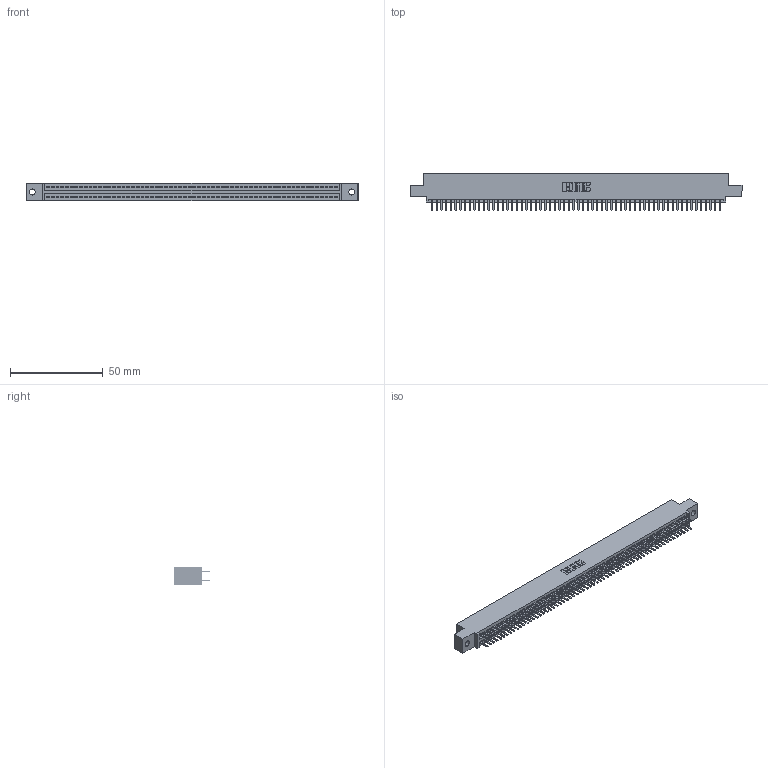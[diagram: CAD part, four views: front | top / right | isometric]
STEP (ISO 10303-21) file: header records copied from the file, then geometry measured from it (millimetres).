
FILE_DESCRIPTION (( 'STEP AP203' ), '1' );
FILE_NAME ('395-124-520-502.STEP', '2018-12-03T21:40:19', ( '' ), ( '' ), 'SwSTEP 2.0', 'SolidWorks 2016', '' );
FILE_SCHEMA (( 'CONFIG_CONTROL_DESIGN' ));
Length unit declared in the file: inch
Products named in the file (3): 395-124-520-502; 345-292-001_345-293-120; 345 Part_0.110 Offset - 0.128 Dia
Assembly tree (125 placements, depth 2):
  395-124-520-502
    345 Part_0.110 Offset - 0.128 Dia
    345-292-001_345-293-120  x124
Bounding box: 178.69 x 19.68 x 9.4 mm (x, y, z)
Volume: 17379.1 mm3; surface area: 25780.8 mm2
Topology: 125 solids, 125 shells, 6826 faces, 19821 edges, 12882 vertices
Faces by surface type: plane 4424, cylinder 2402
Entity records: 46203 total; most frequent: CARTESIAN_POINT 7740, ORIENTED_EDGE 7662, DIRECTION 6787, EDGE_CURVE 3831, LINE 3447, VECTOR 3447, VERTEX_POINT 2550, AXIS2_PLACEMENT_3D 1670
